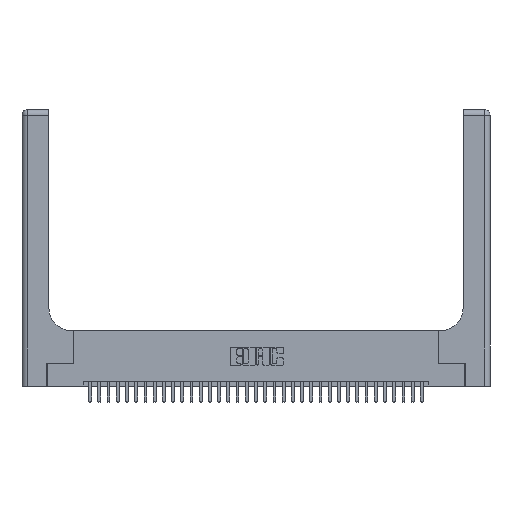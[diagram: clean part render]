
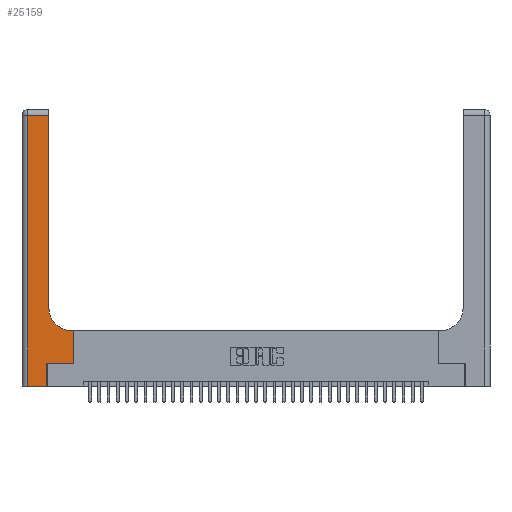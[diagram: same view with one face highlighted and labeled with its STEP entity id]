
A CAD part, top view. The second image highlights one B-rep face of the part: STEP entity #25159.
In plain terms, the highlighted planar face has unit normal (0, 0, 1).
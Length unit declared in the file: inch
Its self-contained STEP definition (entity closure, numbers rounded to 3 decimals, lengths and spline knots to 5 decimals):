
#1248 = EDGE_CURVE ( 'NONE', #18965, #25551, #9543, .T. ) ;
#1391 = VERTEX_POINT ( 'NONE', #22009 ) ;
#2453 = PLANE ( 'NONE',  #14922 ) ;
#2818 = AXIS2_PLACEMENT_3D ( 'NONE', #7387, #26233, #10070 ) ;
#3081 = LINE ( 'NONE', #29776, #30968 ) ;
#3136 = ORIENTED_EDGE ( 'NONE', *, *, #20533, .T. ) ;
#3541 = LINE ( 'NONE', #23794, #9076 ) ;
#4002 = CARTESIAN_POINT ( 'NONE',  ( 0.06, 0., 0.37 ) ) ;
#4395 = CARTESIAN_POINT ( 'NONE',  ( 0.06, 2.94, 0.37 ) ) ;
#4661 = VERTEX_POINT ( 'NONE', #4002 ) ;
#5293 = CARTESIAN_POINT ( 'NONE',  ( 0.269, 0.25, 0.37 ) ) ;
#6043 = VECTOR ( 'NONE', #6182, 39.37008 ) ;
#6182 = DIRECTION ( 'NONE',  ( 0., 1., 0. ) ) ;
#6487 = VECTOR ( 'NONE', #24979, 39.37008 ) ;
#6980 = EDGE_CURVE ( 'NONE', #25636, #26750, #34710, .T. ) ;
#7159 = EDGE_CURVE ( 'NONE', #22761, #13432, #16208, .T. ) ;
#7387 = CARTESIAN_POINT ( 'NONE',  ( 0.5415, 0.85, 0.37 ) ) ;
#7600 = LINE ( 'NONE', #32003, #28231 ) ;
#7954 = DIRECTION ( 'NONE',  ( -1., 0., 0. ) ) ;
#9076 = VECTOR ( 'NONE', #10331, 39.37008 ) ;
#9543 = LINE ( 'NONE', #13378, #30181 ) ;
#9887 = EDGE_CURVE ( 'NONE', #1391, #25636, #13230, .T. ) ;
#10070 = DIRECTION ( 'NONE',  ( 1., 0., 0. ) ) ;
#10331 = DIRECTION ( 'NONE',  ( 0., -1., 0. ) ) ;
#10565 = DIRECTION ( 'NONE',  ( 1., 0., 0. ) ) ;
#12143 = ORIENTED_EDGE ( 'NONE', *, *, #17292, .T. ) ;
#12209 = LINE ( 'NONE', #14005, #17761 ) ;
#13230 = LINE ( 'NONE', #16953, #6043 ) ;
#13378 = CARTESIAN_POINT ( 'NONE',  ( 0.5585, 0.25, 0.37 ) ) ;
#13432 = VERTEX_POINT ( 'NONE', #5293 ) ;
#13848 = EDGE_LOOP ( 'NONE', ( #17987, #30147, #30584, #3136, #32685, #19744, #28561, #26897, #12143 ) ) ;
#14005 = CARTESIAN_POINT ( 'NONE',  ( 0.269, 0.25, 0.37 ) ) ;
#14922 = AXIS2_PLACEMENT_3D ( 'NONE', #21411, #24076, #7954 ) ;
#14926 = VERTEX_POINT ( 'NONE', #19771 ) ;
#15004 = CARTESIAN_POINT ( 'NONE',  ( 0.269, 0., 0.37 ) ) ;
#15019 = CARTESIAN_POINT ( 'NONE',  ( 0.5585, 0.6, 0.37 ) ) ;
#16113 = DIRECTION ( 'NONE',  ( 0., 1., 0. ) ) ;
#16208 = LINE ( 'NONE', #16878, #6487 ) ;
#16744 = DIRECTION ( 'NONE',  ( 1., 0., 0. ) ) ;
#16878 = CARTESIAN_POINT ( 'NONE',  ( 0.269, 0., 0.37 ) ) ;
#16953 = CARTESIAN_POINT ( 'NONE',  ( 0.2915, 3., 0.37 ) ) ;
#17292 = EDGE_CURVE ( 'NONE', #14926, #1391, #30509, .T. ) ;
#17761 = VECTOR ( 'NONE', #16744, 39.37008 ) ;
#17987 = ORIENTED_EDGE ( 'NONE', *, *, #9887, .T. ) ;
#18909 = CARTESIAN_POINT ( 'NONE',  ( 0., 2.94, 0.37 ) ) ;
#18965 = VERTEX_POINT ( 'NONE', #33495 ) ;
#19744 = ORIENTED_EDGE ( 'NONE', *, *, #20654, .T. ) ;
#19771 = CARTESIAN_POINT ( 'NONE',  ( 0.5415, 0.6, 0.37 ) ) ;
#20533 = EDGE_CURVE ( 'NONE', #4661, #22761, #7600, .T. ) ;
#20654 = EDGE_CURVE ( 'NONE', #13432, #18965, #12209, .T. ) ;
#21411 = CARTESIAN_POINT ( 'NONE',  ( 0., 3., 0.37 ) ) ;
#21606 = DIRECTION ( 'NONE',  ( -1., 0., 0. ) ) ;
#22009 = CARTESIAN_POINT ( 'NONE',  ( 0.2915, 0.85, 0.37 ) ) ;
#22761 = VERTEX_POINT ( 'NONE', #15004 ) ;
#23794 = CARTESIAN_POINT ( 'NONE',  ( 0.06, 3., 0.37 ) ) ;
#24076 = DIRECTION ( 'NONE',  ( 0., 0., -1. ) ) ;
#24979 = DIRECTION ( 'NONE',  ( 0., 1., 0. ) ) ;
#25159 = ADVANCED_FACE ( 'NONE', ( #27269 ), #2453, .F. ) ;
#25551 = VERTEX_POINT ( 'NONE', #15019 ) ;
#25636 = VERTEX_POINT ( 'NONE', #29253 ) ;
#26233 = DIRECTION ( 'NONE',  ( 0., 0., -1. ) ) ;
#26750 = VERTEX_POINT ( 'NONE', #4395 ) ;
#26897 = ORIENTED_EDGE ( 'NONE', *, *, #30008, .T. ) ;
#27269 = FACE_OUTER_BOUND ( 'NONE', #13848, .T. ) ;
#28231 = VECTOR ( 'NONE', #10565, 39.37008 ) ;
#28561 = ORIENTED_EDGE ( 'NONE', *, *, #1248, .T. ) ;
#29253 = CARTESIAN_POINT ( 'NONE',  ( 0.2915, 2.94, 0.37 ) ) ;
#29776 = CARTESIAN_POINT ( 'NONE',  ( 0.2915, 0.6, 0.37 ) ) ;
#29840 = EDGE_CURVE ( 'NONE', #26750, #4661, #3541, .T. ) ;
#30008 = EDGE_CURVE ( 'NONE', #25551, #14926, #3081, .T. ) ;
#30147 = ORIENTED_EDGE ( 'NONE', *, *, #6980, .T. ) ;
#30181 = VECTOR ( 'NONE', #16113, 39.37008 ) ;
#30509 = CIRCLE ( 'NONE', #2818, 0.25 ) ;
#30584 = ORIENTED_EDGE ( 'NONE', *, *, #29840, .T. ) ;
#30968 = VECTOR ( 'NONE', #32439, 39.37008 ) ;
#32003 = CARTESIAN_POINT ( 'NONE',  ( 0., 0., 0.37 ) ) ;
#32439 = DIRECTION ( 'NONE',  ( -1., 0., 0. ) ) ;
#32685 = ORIENTED_EDGE ( 'NONE', *, *, #7159, .T. ) ;
#33495 = CARTESIAN_POINT ( 'NONE',  ( 0.5585, 0.25, 0.37 ) ) ;
#33876 = VECTOR ( 'NONE', #21606, 39.37008 ) ;
#34710 = LINE ( 'NONE', #18909, #33876 ) ;
